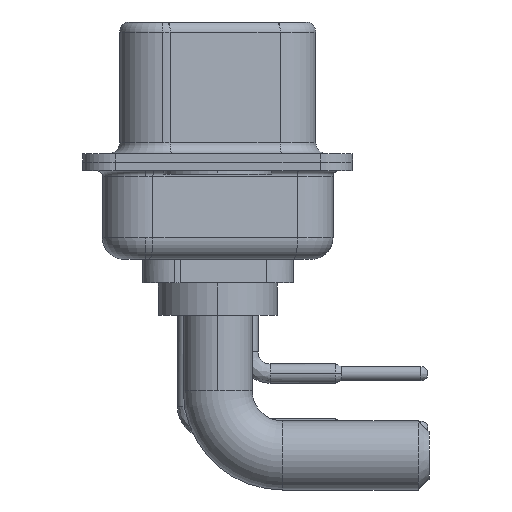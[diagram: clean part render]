
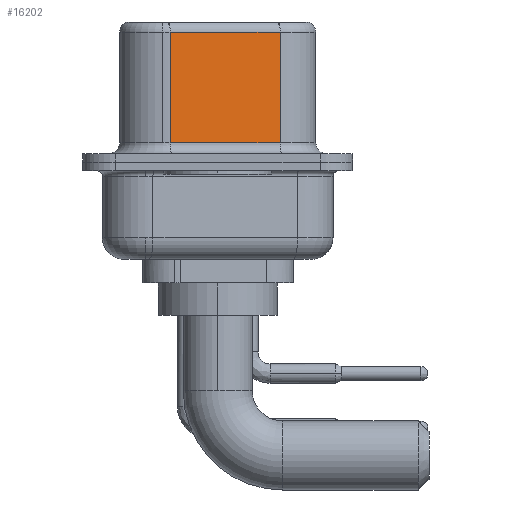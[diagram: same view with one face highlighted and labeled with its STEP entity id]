
A CAD part, left-side view. The second image highlights one B-rep face of the part: STEP entity #16202.
In plain terms, the highlighted planar face has unit normal (-0.985, -0.174, 0).
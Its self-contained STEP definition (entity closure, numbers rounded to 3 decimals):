
#861 = AXIS2_PLACEMENT_3D ( 'NONE', #18011, #11819, #26422 ) ;
#1657 = DIRECTION ( 'NONE',  ( 0., 0., -1. ) ) ;
#2442 = CARTESIAN_POINT ( 'NONE',  ( 3.68, 2.203, 0.9 ) ) ;
#3177 = PLANE ( 'NONE',  #861 ) ;
#3616 = EDGE_CURVE ( 'NONE', #22683, #5264, #26432, .T. ) ;
#5264 = VERTEX_POINT ( 'NONE', #9958 ) ;
#5984 = LINE ( 'NONE', #24240, #6091 ) ;
#6091 = VECTOR ( 'NONE', #1657, 1000. ) ;
#6559 = CARTESIAN_POINT ( 'NONE',  ( 3.68, 2.203, 6.02 ) ) ;
#7372 = EDGE_CURVE ( 'NONE', #12386, #11497, #21514, .T. ) ;
#9958 = CARTESIAN_POINT ( 'NONE',  ( 4.58, -2.897, 0.9 ) ) ;
#11497 = VERTEX_POINT ( 'NONE', #6559 ) ;
#11819 = DIRECTION ( 'NONE',  ( 0.985, 0.174, 0. ) ) ;
#11934 = ORIENTED_EDGE ( 'NONE', *, *, #26483, .F. ) ;
#12386 = VERTEX_POINT ( 'NONE', #12828 ) ;
#12606 = CARTESIAN_POINT ( 'NONE',  ( 4.58, -2.897, 6.52 ) ) ;
#12828 = CARTESIAN_POINT ( 'NONE',  ( 4.58, -2.897, 6.02 ) ) ;
#13978 = CARTESIAN_POINT ( 'NONE',  ( 4.58, -2.897, 0.9 ) ) ;
#15157 = VECTOR ( 'NONE', #16656, 1000. ) ;
#16202 = ADVANCED_FACE ( 'NONE', ( #21675 ), #3177, .F. ) ;
#16656 = DIRECTION ( 'NONE',  ( 0., 0., -1. ) ) ;
#16932 = DIRECTION ( 'NONE',  ( -0.174, 0.985, 0. ) ) ;
#17330 = CARTESIAN_POINT ( 'NONE',  ( 4.58, -2.897, 6.02 ) ) ;
#18011 = CARTESIAN_POINT ( 'NONE',  ( 4.58, -2.897, 6.52 ) ) ;
#18162 = DIRECTION ( 'NONE',  ( 0.174, -0.985, 0. ) ) ;
#18873 = VECTOR ( 'NONE', #18162, 1000. ) ;
#19927 = ORIENTED_EDGE ( 'NONE', *, *, #7372, .T. ) ;
#21514 = LINE ( 'NONE', #17330, #23223 ) ;
#21675 = FACE_OUTER_BOUND ( 'NONE', #21798, .T. ) ;
#21798 = EDGE_LOOP ( 'NONE', ( #11934, #19927, #25848, #24019 ) ) ;
#22683 = VERTEX_POINT ( 'NONE', #2442 ) ;
#23007 = LINE ( 'NONE', #12606, #15157 ) ;
#23223 = VECTOR ( 'NONE', #16932, 1000. ) ;
#24019 = ORIENTED_EDGE ( 'NONE', *, *, #3616, .T. ) ;
#24240 = CARTESIAN_POINT ( 'NONE',  ( 3.68, 2.203, 6.52 ) ) ;
#25848 = ORIENTED_EDGE ( 'NONE', *, *, #26394, .T. ) ;
#26394 = EDGE_CURVE ( 'NONE', #11497, #22683, #5984, .T. ) ;
#26422 = DIRECTION ( 'NONE',  ( -0.174, 0.985, 0. ) ) ;
#26432 = LINE ( 'NONE', #13978, #18873 ) ;
#26483 = EDGE_CURVE ( 'NONE', #12386, #5264, #23007, .T. ) ;
